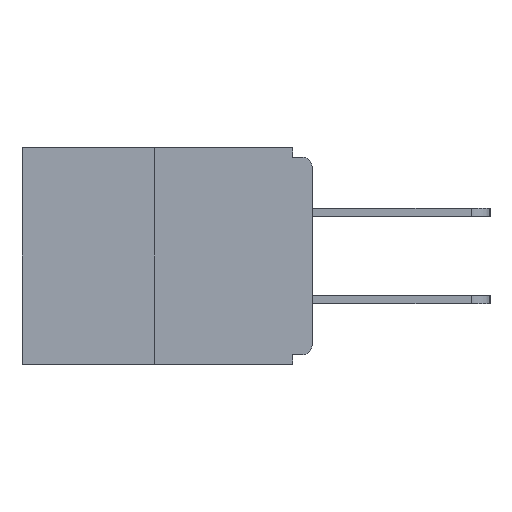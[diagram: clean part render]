
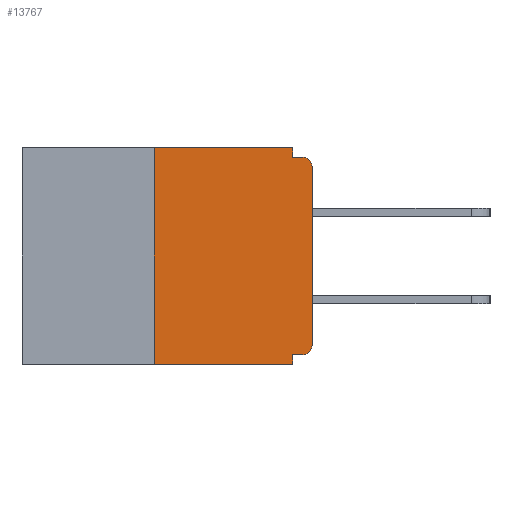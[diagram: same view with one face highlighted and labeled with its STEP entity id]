
A CAD part, left-side view. The second image highlights one B-rep face of the part: STEP entity #13767.
In plain terms, the highlighted planar face has unit normal (-1, 0, 0).
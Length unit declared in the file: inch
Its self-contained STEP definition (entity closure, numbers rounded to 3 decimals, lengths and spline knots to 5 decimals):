
#11 = CARTESIAN_POINT ( 'NONE',  ( 0., 0.015, -0.015 ) ) ;
#387 = CARTESIAN_POINT ( 'NONE',  ( 0., 0.46, -0.343 ) ) ;
#495 = ORIENTED_EDGE ( 'NONE', *, *, #2430, .T. ) ;
#872 = ORIENTED_EDGE ( 'NONE', *, *, #8662, .F. ) ;
#1048 = EDGE_CURVE ( 'NONE', #4875, #2999, #24784, .T. ) ;
#1281 = DIRECTION ( 'NONE',  ( 0., -1., 0. ) ) ;
#1664 = EDGE_CURVE ( 'NONE', #4791, #6608, #8338, .T. ) ;
#2078 = EDGE_CURVE ( 'NONE', #28368, #2999, #5599, .T. ) ;
#2430 = EDGE_CURVE ( 'NONE', #30357, #18739, #11379, .T. ) ;
#2957 = VECTOR ( 'NONE', #7820, 39.37008 ) ;
#2999 = VERTEX_POINT ( 'NONE', #13322 ) ;
#3026 = DIRECTION ( 'NONE',  ( 0., 0., -1. ) ) ;
#3509 = PLANE ( 'NONE',  #29908 ) ;
#4141 = DIRECTION ( 'NONE',  ( 0., 0., -1. ) ) ;
#4193 = CARTESIAN_POINT ( 'NONE',  ( 0., 0.015, -0.03 ) ) ;
#4298 = LINE ( 'NONE', #13707, #25411 ) ;
#4791 = VERTEX_POINT ( 'NONE', #13418 ) ;
#4875 = VERTEX_POINT ( 'NONE', #11809 ) ;
#5190 = CARTESIAN_POINT ( 'NONE',  ( 0., 0., -0.313 ) ) ;
#5391 = VERTEX_POINT ( 'NONE', #16087 ) ;
#5396 = CARTESIAN_POINT ( 'NONE',  ( 0., 0.015, -0.313 ) ) ;
#5599 = LINE ( 'NONE', #28084, #16959 ) ;
#5847 = DIRECTION ( 'NONE',  ( 0., 1., 0. ) ) ;
#6065 = CARTESIAN_POINT ( 'NONE',  ( 0., 0.46, 0. ) ) ;
#6172 = LINE ( 'NONE', #25447, #29982 ) ;
#6608 = VERTEX_POINT ( 'NONE', #11 ) ;
#7804 = ORIENTED_EDGE ( 'NONE', *, *, #21298, .F. ) ;
#7820 = DIRECTION ( 'NONE',  ( 0., 0., 1. ) ) ;
#8294 = DIRECTION ( 'NONE',  ( 1., 0., 0. ) ) ;
#8338 = CIRCLE ( 'NONE', #20037, 0.015 ) ;
#8662 = EDGE_CURVE ( 'NONE', #4875, #5391, #17236, .T. ) ;
#8806 = ORIENTED_EDGE ( 'NONE', *, *, #1048, .T. ) ;
#8838 = VECTOR ( 'NONE', #10430, 39.37008 ) ;
#9419 = ORIENTED_EDGE ( 'NONE', *, *, #1664, .T. ) ;
#9744 = CARTESIAN_POINT ( 'NONE',  ( 0., 0.25, 0. ) ) ;
#10277 = CARTESIAN_POINT ( 'NONE',  ( 0., 0.015, -0.328 ) ) ;
#10430 = DIRECTION ( 'NONE',  ( 0., -1., 0. ) ) ;
#11379 = CIRCLE ( 'NONE', #20518, 0.015 ) ;
#11809 = CARTESIAN_POINT ( 'NONE',  ( 0., 0.25, -0.343 ) ) ;
#12431 = ORIENTED_EDGE ( 'NONE', *, *, #23348, .T. ) ;
#12834 = VECTOR ( 'NONE', #23283, 39.37008 ) ;
#13322 = CARTESIAN_POINT ( 'NONE',  ( 0., 0.031, -0.343 ) ) ;
#13418 = CARTESIAN_POINT ( 'NONE',  ( 0., 0., -0.03 ) ) ;
#13707 = CARTESIAN_POINT ( 'NONE',  ( 0., 0.031, 0. ) ) ;
#13767 = ADVANCED_FACE ( 'NONE', ( #22610 ), #3509, .F. ) ;
#13918 = DIRECTION ( 'NONE',  ( 0., 0., -1. ) ) ;
#14816 = VECTOR ( 'NONE', #1281, 39.37008 ) ;
#15946 = LINE ( 'NONE', #25677, #14816 ) ;
#16087 = CARTESIAN_POINT ( 'NONE',  ( 0., 0.25, 0. ) ) ;
#16319 = VECTOR ( 'NONE', #25107, 39.37008 ) ;
#16959 = VECTOR ( 'NONE', #27446, 39.37008 ) ;
#17236 = LINE ( 'NONE', #9744, #2957 ) ;
#17335 = VERTEX_POINT ( 'NONE', #24040 ) ;
#17447 = ORIENTED_EDGE ( 'NONE', *, *, #27110, .F. ) ;
#18289 = EDGE_LOOP ( 'NONE', ( #28923, #872, #8806, #20612, #7804, #495, #12431, #9419, #17447, #19719 ) ) ;
#18739 = VERTEX_POINT ( 'NONE', #5190 ) ;
#19719 = ORIENTED_EDGE ( 'NONE', *, *, #22124, .F. ) ;
#20037 = AXIS2_PLACEMENT_3D ( 'NONE', #4193, #26495, #13918 ) ;
#20518 = AXIS2_PLACEMENT_3D ( 'NONE', #5396, #24383, #24220 ) ;
#20612 = ORIENTED_EDGE ( 'NONE', *, *, #2078, .F. ) ;
#20647 = LINE ( 'NONE', #30386, #16319 ) ;
#20665 = VERTEX_POINT ( 'NONE', #28191 ) ;
#20728 = CARTESIAN_POINT ( 'NONE',  ( 0., 0.031, -0.328 ) ) ;
#21298 = EDGE_CURVE ( 'NONE', #30357, #28368, #6172, .T. ) ;
#21769 = LINE ( 'NONE', #26148, #12834 ) ;
#22124 = EDGE_CURVE ( 'NONE', #17335, #20665, #4298, .T. ) ;
#22610 = FACE_OUTER_BOUND ( 'NONE', #18289, .T. ) ;
#23283 = DIRECTION ( 'NONE',  ( 0., -1., 0. ) ) ;
#23348 = EDGE_CURVE ( 'NONE', #18739, #4791, #20647, .T. ) ;
#24040 = CARTESIAN_POINT ( 'NONE',  ( 0., 0.031, 0. ) ) ;
#24220 = DIRECTION ( 'NONE',  ( 0., 0., -1. ) ) ;
#24383 = DIRECTION ( 'NONE',  ( -1., 0., 0. ) ) ;
#24784 = LINE ( 'NONE', #387, #8838 ) ;
#25107 = DIRECTION ( 'NONE',  ( 0., 0., 1. ) ) ;
#25411 = VECTOR ( 'NONE', #4141, 39.37008 ) ;
#25447 = CARTESIAN_POINT ( 'NONE',  ( 0., 0., -0.328 ) ) ;
#25677 = CARTESIAN_POINT ( 'NONE',  ( 0., 0.46, 0. ) ) ;
#26148 = CARTESIAN_POINT ( 'NONE',  ( 0., 0., -0.015 ) ) ;
#26495 = DIRECTION ( 'NONE',  ( -1., 0., 0. ) ) ;
#27110 = EDGE_CURVE ( 'NONE', #20665, #6608, #21769, .T. ) ;
#27446 = DIRECTION ( 'NONE',  ( 0., 0., -1. ) ) ;
#28084 = CARTESIAN_POINT ( 'NONE',  ( 0., 0.031, -0.343 ) ) ;
#28191 = CARTESIAN_POINT ( 'NONE',  ( 0., 0.031, -0.015 ) ) ;
#28299 = EDGE_CURVE ( 'NONE', #5391, #17335, #15946, .T. ) ;
#28368 = VERTEX_POINT ( 'NONE', #20728 ) ;
#28923 = ORIENTED_EDGE ( 'NONE', *, *, #28299, .F. ) ;
#29908 = AXIS2_PLACEMENT_3D ( 'NONE', #6065, #8294, #3026 ) ;
#29982 = VECTOR ( 'NONE', #5847, 39.37008 ) ;
#30357 = VERTEX_POINT ( 'NONE', #10277 ) ;
#30386 = CARTESIAN_POINT ( 'NONE',  ( 0., 0., 0. ) ) ;
